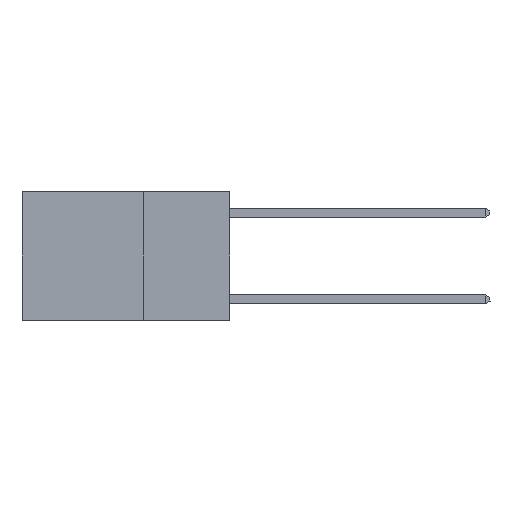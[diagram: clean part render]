
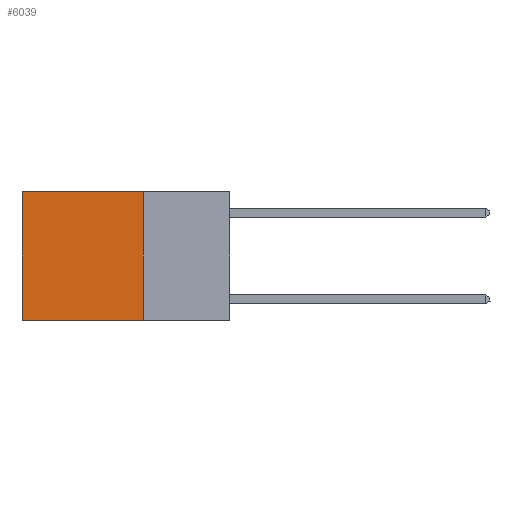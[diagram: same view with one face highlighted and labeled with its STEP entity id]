
A CAD part, left-side view. The second image highlights one B-rep face of the part: STEP entity #6039.
In plain terms, the highlighted planar face has unit normal (-1, 0, 0).
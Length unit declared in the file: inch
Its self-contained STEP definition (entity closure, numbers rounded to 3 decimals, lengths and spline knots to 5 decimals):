
#237 = VECTOR ( 'NONE', #704, 39.37008 ) ;
#704 = DIRECTION ( 'NONE',  ( 0., 0., -1. ) ) ;
#1251 = DIRECTION ( 'NONE',  ( 0., 0., -1. ) ) ;
#1371 = ORIENTED_EDGE ( 'NONE', *, *, #7408, .T. ) ;
#1631 = AXIS2_PLACEMENT_3D ( 'NONE', #6925, #8060, #1251 ) ;
#1965 = EDGE_CURVE ( 'NONE', #9511, #9753, #6335, .T. ) ;
#2110 = CARTESIAN_POINT ( 'NONE',  ( 0.2625, 0.25, 0. ) ) ;
#2358 = DIRECTION ( 'NONE',  ( 0., 1., 0. ) ) ;
#2823 = DIRECTION ( 'NONE',  ( 0., 1., 0. ) ) ;
#3616 = VERTEX_POINT ( 'NONE', #12541 ) ;
#3819 = VECTOR ( 'NONE', #2358, 39.37008 ) ;
#5300 = ORIENTED_EDGE ( 'NONE', *, *, #7254, .F. ) ;
#6039 = ADVANCED_FACE ( 'NONE', ( #13635 ), #13555, .F. ) ;
#6141 = LINE ( 'NONE', #9172, #3819 ) ;
#6335 = LINE ( 'NONE', #14131, #237 ) ;
#6336 = LINE ( 'NONE', #12866, #11931 ) ;
#6925 = CARTESIAN_POINT ( 'NONE',  ( 0.2625, 0.25, 0. ) ) ;
#7254 = EDGE_CURVE ( 'NONE', #12453, #3616, #8270, .T. ) ;
#7408 = EDGE_CURVE ( 'NONE', #12453, #9511, #6141, .T. ) ;
#7861 = EDGE_CURVE ( 'NONE', #3616, #9753, #6336, .T. ) ;
#8060 = DIRECTION ( 'NONE',  ( 1., 0., 0. ) ) ;
#8077 = EDGE_LOOP ( 'NONE', ( #11568, #10286, #5300, #1371 ) ) ;
#8270 = LINE ( 'NONE', #2110, #10895 ) ;
#8776 = CARTESIAN_POINT ( 'NONE',  ( 0.2625, 0.25, 0. ) ) ;
#9172 = CARTESIAN_POINT ( 'NONE',  ( 0.2625, 0.25, 0. ) ) ;
#9176 = CARTESIAN_POINT ( 'NONE',  ( 0.2625, 0.6, 0. ) ) ;
#9511 = VERTEX_POINT ( 'NONE', #9176 ) ;
#9753 = VERTEX_POINT ( 'NONE', #12733 ) ;
#10063 = DIRECTION ( 'NONE',  ( 0., 0., -1. ) ) ;
#10286 = ORIENTED_EDGE ( 'NONE', *, *, #7861, .F. ) ;
#10895 = VECTOR ( 'NONE', #10063, 39.37008 ) ;
#11568 = ORIENTED_EDGE ( 'NONE', *, *, #1965, .T. ) ;
#11931 = VECTOR ( 'NONE', #2823, 39.37008 ) ;
#12453 = VERTEX_POINT ( 'NONE', #8776 ) ;
#12541 = CARTESIAN_POINT ( 'NONE',  ( 0.2625, 0.25, -0.37 ) ) ;
#12733 = CARTESIAN_POINT ( 'NONE',  ( 0.2625, 0.6, -0.37 ) ) ;
#12866 = CARTESIAN_POINT ( 'NONE',  ( 0.2625, 0.25, -0.37 ) ) ;
#13555 = PLANE ( 'NONE',  #1631 ) ;
#13635 = FACE_OUTER_BOUND ( 'NONE', #8077, .T. ) ;
#14131 = CARTESIAN_POINT ( 'NONE',  ( 0.2625, 0.6, 0. ) ) ;
